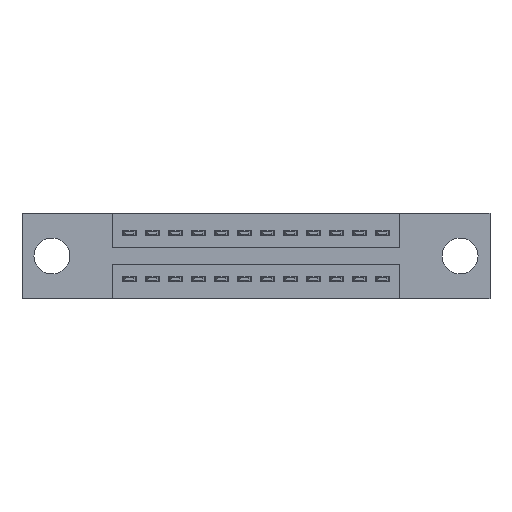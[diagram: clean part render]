
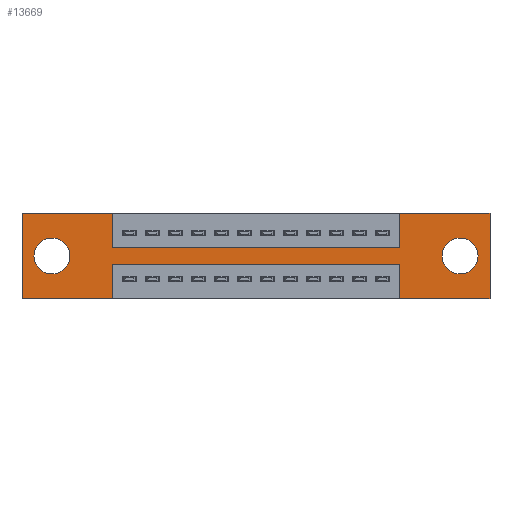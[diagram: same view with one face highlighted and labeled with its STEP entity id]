
A CAD part, front view. The second image highlights one B-rep face of the part: STEP entity #13669.
In plain terms, the highlighted planar face has unit normal (0, -1, 0).
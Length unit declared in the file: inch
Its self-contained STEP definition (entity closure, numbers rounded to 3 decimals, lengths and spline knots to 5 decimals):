
#303 = VECTOR ( 'NONE', #717, 39.37008 ) ;
#346 = ORIENTED_EDGE ( 'NONE', *, *, #5781, .F. ) ;
#531 = CARTESIAN_POINT ( 'NONE',  ( 2.035, 0., -0.37 ) ) ;
#560 = CARTESIAN_POINT ( 'NONE',  ( 1.6425, 0., 0. ) ) ;
#717 = DIRECTION ( 'NONE',  ( -1., 0., 0. ) ) ;
#832 = DIRECTION ( 'NONE',  ( 0., 0., 1. ) ) ;
#848 = LINE ( 'NONE', #7276, #5374 ) ;
#851 = VERTEX_POINT ( 'NONE', #3751 ) ;
#954 = DIRECTION ( 'NONE',  ( 0., 1., 0. ) ) ;
#1130 = ORIENTED_EDGE ( 'NONE', *, *, #2852, .T. ) ;
#1188 = DIRECTION ( 'NONE',  ( 1., 0., 0. ) ) ;
#1192 = LINE ( 'NONE', #3266, #5034 ) ;
#1404 = AXIS2_PLACEMENT_3D ( 'NONE', #7290, #4305, #2028 ) ;
#1504 = DIRECTION ( 'NONE',  ( 0., 0., -1. ) ) ;
#1733 = DIRECTION ( 'NONE',  ( 0., 0., 1. ) ) ;
#1905 = DIRECTION ( 'NONE',  ( 0., 1., 0. ) ) ;
#2023 = LINE ( 'NONE', #9257, #4546 ) ;
#2028 = DIRECTION ( 'NONE',  ( 0., 0., 1. ) ) ;
#2113 = CIRCLE ( 'NONE', #5035, 0.078 ) ;
#2171 = DIRECTION ( 'NONE',  ( 0., 0., 1. ) ) ;
#2219 = VERTEX_POINT ( 'NONE', #4385 ) ;
#2226 = CARTESIAN_POINT ( 'NONE',  ( 0.3925, 0., -0.37 ) ) ;
#2402 = VERTEX_POINT ( 'NONE', #12016 ) ;
#2425 = VERTEX_POINT ( 'NONE', #9310 ) ;
#2492 = CARTESIAN_POINT ( 'NONE',  ( 0.3925, 0., 0. ) ) ;
#2517 = VECTOR ( 'NONE', #5150, 39.37008 ) ;
#2621 = ORIENTED_EDGE ( 'NONE', *, *, #8896, .F. ) ;
#2852 = EDGE_CURVE ( 'NONE', #10102, #5183, #5669, .T. ) ;
#2882 = EDGE_CURVE ( 'NONE', #10136, #2219, #7054, .T. ) ;
#2910 = DIRECTION ( 'NONE',  ( 0., 0., 1. ) ) ;
#2992 = VECTOR ( 'NONE', #1188, 39.37008 ) ;
#3083 = EDGE_CURVE ( 'NONE', #5320, #4698, #8438, .T. ) ;
#3266 = CARTESIAN_POINT ( 'NONE',  ( 0., 0., 0. ) ) ;
#3323 = FACE_BOUND ( 'NONE', #10215, .T. ) ;
#3379 = EDGE_CURVE ( 'NONE', #2219, #6531, #12528, .T. ) ;
#3389 = DIRECTION ( 'NONE',  ( 0., -1., 0. ) ) ;
#3390 = CARTESIAN_POINT ( 'NONE',  ( 2.035, 0., 0. ) ) ;
#3582 = VERTEX_POINT ( 'NONE', #6804 ) ;
#3688 = VECTOR ( 'NONE', #13568, 39.37008 ) ;
#3692 = VECTOR ( 'NONE', #5027, 39.37008 ) ;
#3751 = CARTESIAN_POINT ( 'NONE',  ( 0.13, 0., -0.263 ) ) ;
#3916 = LINE ( 'NONE', #13438, #6348 ) ;
#4110 = CIRCLE ( 'NONE', #9447, 0.078 ) ;
#4128 = CARTESIAN_POINT ( 'NONE',  ( 0.3925, 0., 0. ) ) ;
#4140 = ORIENTED_EDGE ( 'NONE', *, *, #5950, .T. ) ;
#4305 = DIRECTION ( 'NONE',  ( 0., 1., 0. ) ) ;
#4375 = CARTESIAN_POINT ( 'NONE',  ( 0., 0., 0. ) ) ;
#4385 = CARTESIAN_POINT ( 'NONE',  ( 1.6425, 0., 0. ) ) ;
#4546 = VECTOR ( 'NONE', #2910, 39.37008 ) ;
#4698 = VERTEX_POINT ( 'NONE', #11359 ) ;
#4769 = DIRECTION ( 'NONE',  ( 0., 1., 0. ) ) ;
#4779 = EDGE_CURVE ( 'NONE', #6765, #8212, #13654, .T. ) ;
#4855 = EDGE_LOOP ( 'NONE', ( #346, #11328, #12030, #2621, #13353, #8589, #13308, #5254, #8213, #9082, #6688, #5752 ) ) ;
#4889 = ORIENTED_EDGE ( 'NONE', *, *, #9102, .T. ) ;
#5027 = DIRECTION ( 'NONE',  ( 1., 0., 0. ) ) ;
#5034 = VECTOR ( 'NONE', #2171, 39.37008 ) ;
#5035 = AXIS2_PLACEMENT_3D ( 'NONE', #11107, #954, #832 ) ;
#5056 = DIRECTION ( 'NONE',  ( 0., 0., -1. ) ) ;
#5114 = DIRECTION ( 'NONE',  ( -1., 0., 0. ) ) ;
#5150 = DIRECTION ( 'NONE',  ( 1., 0., 0. ) ) ;
#5183 = VERTEX_POINT ( 'NONE', #6238 ) ;
#5254 = ORIENTED_EDGE ( 'NONE', *, *, #11813, .F. ) ;
#5253 = CARTESIAN_POINT ( 'NONE',  ( 0.13, 0., -0.107 ) ) ;
#5320 = VERTEX_POINT ( 'NONE', #2226 ) ;
#5356 = EDGE_CURVE ( 'NONE', #851, #9738, #2113, .T. ) ;
#5374 = VECTOR ( 'NONE', #11384, 39.37008 ) ;
#5427 = AXIS2_PLACEMENT_3D ( 'NONE', #12917, #3389, #11947 ) ;
#5669 = CIRCLE ( 'NONE', #10772, 0.078 ) ;
#5752 = ORIENTED_EDGE ( 'NONE', *, *, #3083, .F. ) ;
#5781 = EDGE_CURVE ( 'NONE', #2425, #5320, #3916, .T. ) ;
#5945 = VERTEX_POINT ( 'NONE', #13509 ) ;
#5950 = EDGE_CURVE ( 'NONE', #5183, #10102, #4110, .T. ) ;
#6156 = CARTESIAN_POINT ( 'NONE',  ( 0., 0., -0.37 ) ) ;
#6238 = CARTESIAN_POINT ( 'NONE',  ( 1.905, 0., -0.107 ) ) ;
#6348 = VECTOR ( 'NONE', #1504, 39.37008 ) ;
#6438 = FACE_OUTER_BOUND ( 'NONE', #4855, .T. ) ;
#6531 = VERTEX_POINT ( 'NONE', #3390 ) ;
#6688 = ORIENTED_EDGE ( 'NONE', *, *, #7921, .F. ) ;
#6765 = VERTEX_POINT ( 'NONE', #2492 ) ;
#6804 = CARTESIAN_POINT ( 'NONE',  ( 1.6425, 0., -0.37 ) ) ;
#6983 = ORIENTED_EDGE ( 'NONE', *, *, #5356, .T. ) ;
#7054 = LINE ( 'NONE', #560, #13232 ) ;
#7090 = CARTESIAN_POINT ( 'NONE',  ( 0., 0., 0. ) ) ;
#7183 = VERTEX_POINT ( 'NONE', #531 ) ;
#7276 = CARTESIAN_POINT ( 'NONE',  ( 0.3925, 0., -0.22 ) ) ;
#7290 = CARTESIAN_POINT ( 'NONE',  ( 0.13, 0., -0.185 ) ) ;
#7302 = CARTESIAN_POINT ( 'NONE',  ( 1.905, 0., -0.185 ) ) ;
#7360 = EDGE_CURVE ( 'NONE', #6531, #7183, #9331, .T. ) ;
#7622 = LINE ( 'NONE', #4375, #2992 ) ;
#7921 = EDGE_CURVE ( 'NONE', #4698, #2402, #1192, .T. ) ;
#8212 = VERTEX_POINT ( 'NONE', #8313 ) ;
#8213 = ORIENTED_EDGE ( 'NONE', *, *, #4779, .F. ) ;
#8275 = DIRECTION ( 'NONE',  ( 0., 0., -1. ) ) ;
#8313 = CARTESIAN_POINT ( 'NONE',  ( 0.3925, 0., -0.15 ) ) ;
#8438 = LINE ( 'NONE', #6156, #10350 ) ;
#8499 = DIRECTION ( 'NONE',  ( 0., 0., -1. ) ) ;
#8589 = ORIENTED_EDGE ( 'NONE', *, *, #3379, .F. ) ;
#8864 = LINE ( 'NONE', #10930, #303 ) ;
#8896 = EDGE_CURVE ( 'NONE', #7183, #3582, #8864, .T. ) ;
#9025 = CARTESIAN_POINT ( 'NONE',  ( 1.905, 0., -0.185 ) ) ;
#9082 = ORIENTED_EDGE ( 'NONE', *, *, #12019, .F. ) ;
#9102 = EDGE_CURVE ( 'NONE', #9738, #851, #10052, .T. ) ;
#9257 = CARTESIAN_POINT ( 'NONE',  ( 1.6425, 0., -0.37 ) ) ;
#9310 = CARTESIAN_POINT ( 'NONE',  ( 0.3925, 0., -0.22 ) ) ;
#9331 = LINE ( 'NONE', #11704, #3688 ) ;
#9391 = EDGE_LOOP ( 'NONE', ( #4889, #6983 ) ) ;
#9410 = CARTESIAN_POINT ( 'NONE',  ( 1.6425, 0., -0.15 ) ) ;
#9447 = AXIS2_PLACEMENT_3D ( 'NONE', #7302, #1905, #8275 ) ;
#9473 = EDGE_CURVE ( 'NONE', #5945, #2425, #848, .T. ) ;
#9738 = VERTEX_POINT ( 'NONE', #5253 ) ;
#10052 = CIRCLE ( 'NONE', #1404, 0.078 ) ;
#10102 = VERTEX_POINT ( 'NONE', #10249 ) ;
#10130 = VECTOR ( 'NONE', #8499, 39.37008 ) ;
#10136 = VERTEX_POINT ( 'NONE', #9410 ) ;
#10215 = EDGE_LOOP ( 'NONE', ( #4140, #1130 ) ) ;
#10249 = CARTESIAN_POINT ( 'NONE',  ( 1.905, 0., -0.263 ) ) ;
#10350 = VECTOR ( 'NONE', #5114, 39.37008 ) ;
#10586 = CARTESIAN_POINT ( 'NONE',  ( 0.3925, 0., -0.15 ) ) ;
#10772 = AXIS2_PLACEMENT_3D ( 'NONE', #9025, #4769, #5056 ) ;
#10835 = FACE_BOUND ( 'NONE', #9391, .T. ) ;
#10930 = CARTESIAN_POINT ( 'NONE',  ( 0., 0., -0.37 ) ) ;
#11107 = CARTESIAN_POINT ( 'NONE',  ( 0.13, 0., -0.185 ) ) ;
#11328 = ORIENTED_EDGE ( 'NONE', *, *, #9473, .F. ) ;
#11359 = CARTESIAN_POINT ( 'NONE',  ( 0., 0., -0.37 ) ) ;
#11384 = DIRECTION ( 'NONE',  ( -1., 0., 0. ) ) ;
#11704 = CARTESIAN_POINT ( 'NONE',  ( 2.035, 0., 0. ) ) ;
#11748 = PLANE ( 'NONE',  #5427 ) ;
#11813 = EDGE_CURVE ( 'NONE', #8212, #10136, #12731, .T. ) ;
#11947 = DIRECTION ( 'NONE',  ( 0., 0., -1. ) ) ;
#12016 = CARTESIAN_POINT ( 'NONE',  ( 0., 0., 0. ) ) ;
#12019 = EDGE_CURVE ( 'NONE', #2402, #6765, #7622, .T. ) ;
#12030 = ORIENTED_EDGE ( 'NONE', *, *, #13529, .F. ) ;
#12528 = LINE ( 'NONE', #7090, #3692 ) ;
#12731 = LINE ( 'NONE', #10586, #2517 ) ;
#12917 = CARTESIAN_POINT ( 'NONE',  ( 0., 0., -0.37 ) ) ;
#13232 = VECTOR ( 'NONE', #1733, 39.37008 ) ;
#13308 = ORIENTED_EDGE ( 'NONE', *, *, #2882, .F. ) ;
#13353 = ORIENTED_EDGE ( 'NONE', *, *, #7360, .F. ) ;
#13438 = CARTESIAN_POINT ( 'NONE',  ( 0.3925, 0., -0.37 ) ) ;
#13509 = CARTESIAN_POINT ( 'NONE',  ( 1.6425, 0., -0.22 ) ) ;
#13529 = EDGE_CURVE ( 'NONE', #3582, #5945, #2023, .T. ) ;
#13568 = DIRECTION ( 'NONE',  ( 0., 0., -1. ) ) ;
#13654 = LINE ( 'NONE', #4128, #10130 ) ;
#13669 = ADVANCED_FACE ( 'NONE', ( #3323, #10835, #6438 ), #11748, .T. ) ;
